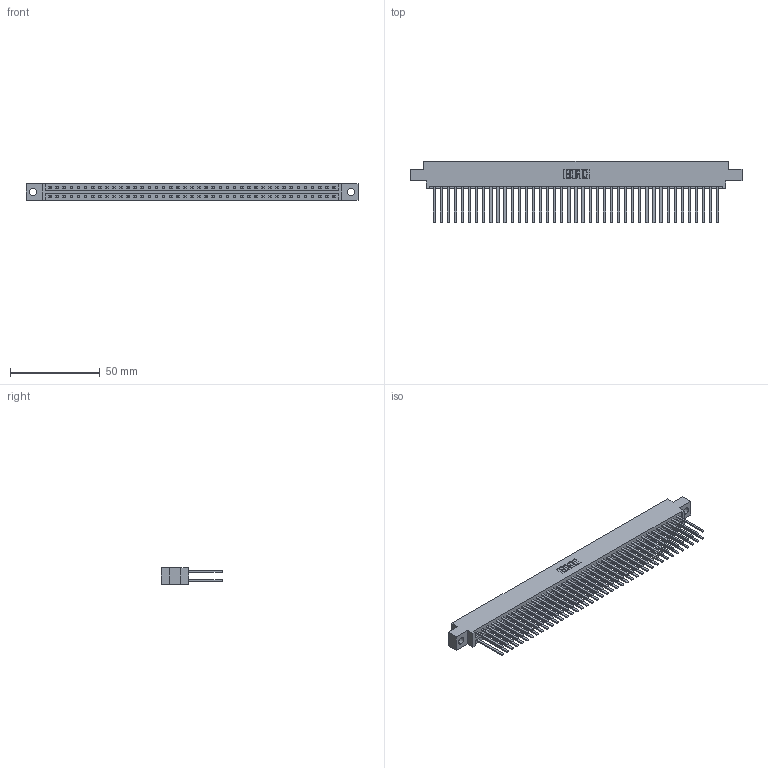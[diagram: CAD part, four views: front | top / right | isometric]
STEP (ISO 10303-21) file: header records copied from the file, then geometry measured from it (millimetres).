
FILE_DESCRIPTION (( 'STEP AP203' ), '1' );
FILE_NAME ('387-082-544-804.STEP', '2018-09-23T20:33:40', ( '' ), ( '' ), 'SwSTEP 2.0', 'SolidWorks 2016', '' );
FILE_SCHEMA (( 'CONFIG_CONTROL_DESIGN' ));
Length unit declared in the file: inch
Products named in the file (3): 337 Part_0.170 Offset - 0.156 Dia-TH; 345-292-001_345-293-144; 387-082-544-804
Assembly tree (83 placements, depth 2):
  387-082-544-804
    337 Part_0.170 Offset - 0.156 Dia-TH
    345-292-001_345-293-144  x82
Bounding box: 185.47 x 34.3 x 9.4 mm (x, y, z)
Volume: 20477.2 mm3; surface area: 26800.1 mm2
Topology: 83 solids, 83 shells, 4054 faces, 12049 edges, 7922 vertices
Faces by surface type: plane 2862, cylinder 1192
Entity records: 31869 total; most frequent: CARTESIAN_POINT 5370, ORIENTED_EDGE 5306, DIRECTION 4565, EDGE_CURVE 2653, VECTOR 2529, LINE 2529, VERTEX_POINT 1766, AXIS2_PLACEMENT_3D 1018
